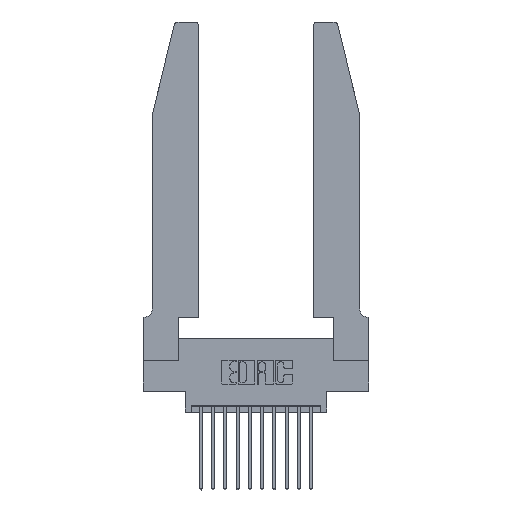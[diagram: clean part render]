
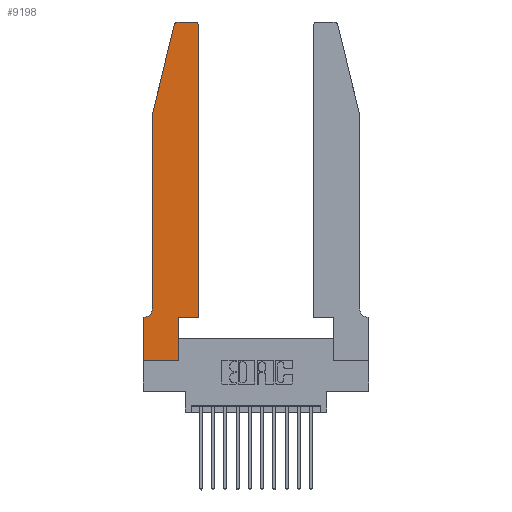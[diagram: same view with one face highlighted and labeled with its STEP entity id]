
A CAD part, top view. The second image highlights one B-rep face of the part: STEP entity #9198.
In plain terms, the highlighted planar face has unit normal (0, 0, 1).
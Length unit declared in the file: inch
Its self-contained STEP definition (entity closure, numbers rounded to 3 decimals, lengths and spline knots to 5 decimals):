
#285 = CARTESIAN_POINT ( 'NONE',  ( 0.284, 2.72, 0.37 ) ) ;
#491 = CARTESIAN_POINT ( 'NONE',  ( 0.2605, 2.75, 0.37 ) ) ;
#730 = CIRCLE ( 'NONE', #12264, 0.03 ) ;
#994 = CARTESIAN_POINT ( 'NONE',  ( 0.0755, 2., 0.37 ) ) ;
#1283 = EDGE_CURVE ( 'NONE', #11578, #4585, #10848, .T. ) ;
#1331 = CARTESIAN_POINT ( 'NONE',  ( 0.284, 2.75, 0.37 ) ) ;
#1340 = CIRCLE ( 'NONE', #5759, 0.07 ) ;
#1403 = VERTEX_POINT ( 'NONE', #15737 ) ;
#1602 = DIRECTION ( 'NONE',  ( 1., 0., 0. ) ) ;
#1617 = EDGE_CURVE ( 'NONE', #6264, #10600, #730, .T. ) ;
#1886 = ORIENTED_EDGE ( 'NONE', *, *, #4167, .T. ) ;
#1912 = LINE ( 'NONE', #8963, #12431 ) ;
#2145 = EDGE_CURVE ( 'NONE', #4585, #13388, #1340, .T. ) ;
#2500 = DIRECTION ( 'NONE',  ( -0.239, -0.971, 0. ) ) ;
#2505 = ORIENTED_EDGE ( 'NONE', *, *, #2699, .T. ) ;
#2699 = EDGE_CURVE ( 'NONE', #11066, #11127, #12644, .T. ) ;
#2708 = DIRECTION ( 'NONE',  ( 0., -1., 0. ) ) ;
#2823 = CARTESIAN_POINT ( 'NONE',  ( 0.4205, 2.75, 0.37 ) ) ;
#3012 = VECTOR ( 'NONE', #8688, 39.37008 ) ;
#3456 = DIRECTION ( 'NONE',  ( 1., 0., 0. ) ) ;
#3475 = CARTESIAN_POINT ( 'NONE',  ( 0.4205, 2.72, 0.37 ) ) ;
#3590 = DIRECTION ( 'NONE',  ( 0., 0., 1. ) ) ;
#4015 = EDGE_CURVE ( 'NONE', #1403, #5739, #5811, .T. ) ;
#4167 = EDGE_CURVE ( 'NONE', #10600, #11578, #1912, .T. ) ;
#4585 = VERTEX_POINT ( 'NONE', #6117 ) ;
#4599 = EDGE_CURVE ( 'NONE', #16292, #9981, #14475, .T. ) ;
#4806 = DIRECTION ( 'NONE',  ( 0., 0., -1. ) ) ;
#5260 = FACE_OUTER_BOUND ( 'NONE', #16275, .T. ) ;
#5327 = CARTESIAN_POINT ( 'NONE',  ( 0.0755, 0.35, 0.37 ) ) ;
#5358 = AXIS2_PLACEMENT_3D ( 'NONE', #3475, #3590, #15305 ) ;
#5403 = VECTOR ( 'NONE', #5986, 39.37008 ) ;
#5739 = VERTEX_POINT ( 'NONE', #8305 ) ;
#5759 = AXIS2_PLACEMENT_3D ( 'NONE', #11400, #4806, #10040 ) ;
#5766 = VECTOR ( 'NONE', #12237, 39.37008 ) ;
#5811 = LINE ( 'NONE', #11386, #12211 ) ;
#5820 = CIRCLE ( 'NONE', #5358, 0.03 ) ;
#5929 = DIRECTION ( 'NONE',  ( 1., 0., 0. ) ) ;
#5986 = DIRECTION ( 'NONE',  ( 0., 1., 0. ) ) ;
#6117 = CARTESIAN_POINT ( 'NONE',  ( 0.0755, 0.42, 0.37 ) ) ;
#6166 = PLANE ( 'NONE',  #10211 ) ;
#6233 = VERTEX_POINT ( 'NONE', #2823 ) ;
#6264 = VERTEX_POINT ( 'NONE', #1331 ) ;
#6312 = ORIENTED_EDGE ( 'NONE', *, *, #1617, .T. ) ;
#6498 = EDGE_CURVE ( 'NONE', #9981, #1403, #16035, .T. ) ;
#6626 = DIRECTION ( 'NONE',  ( 0., 1., 0. ) ) ;
#6808 = CARTESIAN_POINT ( 'NONE',  ( 0.2865, 0.35, 0.37 ) ) ;
#7047 = ORIENTED_EDGE ( 'NONE', *, *, #4599, .T. ) ;
#7128 = DIRECTION ( 'NONE',  ( 0., -1., 0. ) ) ;
#7188 = CARTESIAN_POINT ( 'NONE',  ( 0., 0., 0.37 ) ) ;
#7495 = CARTESIAN_POINT ( 'NONE',  ( 0., 0., 0.37 ) ) ;
#8305 = CARTESIAN_POINT ( 'NONE',  ( 0.4505, 2.72, 0.37 ) ) ;
#8359 = ORIENTED_EDGE ( 'NONE', *, *, #4015, .T. ) ;
#8688 = DIRECTION ( 'NONE',  ( 1., 0., 0. ) ) ;
#8821 = CARTESIAN_POINT ( 'NONE',  ( 0.0055, 0.35, 0.37 ) ) ;
#8963 = CARTESIAN_POINT ( 'NONE',  ( 0.0755, 2., 0.37 ) ) ;
#9198 = ADVANCED_FACE ( 'NONE', ( #5260 ), #6166, .T. ) ;
#9345 = CARTESIAN_POINT ( 'NONE',  ( 0., 0., 0.37 ) ) ;
#9489 = DIRECTION ( 'NONE',  ( 0., 0., 1. ) ) ;
#9929 = ORIENTED_EDGE ( 'NONE', *, *, #1283, .T. ) ;
#9981 = VERTEX_POINT ( 'NONE', #13438 ) ;
#10030 = DIRECTION ( 'NONE',  ( 0., 0., 1. ) ) ;
#10040 = DIRECTION ( 'NONE',  ( -1., 0., 0. ) ) ;
#10211 = AXIS2_PLACEMENT_3D ( 'NONE', #11333, #10030, #3456 ) ;
#10441 = LINE ( 'NONE', #5327, #11683 ) ;
#10454 = EDGE_CURVE ( 'NONE', #5739, #6233, #5820, .T. ) ;
#10600 = VERTEX_POINT ( 'NONE', #13426 ) ;
#10695 = ORIENTED_EDGE ( 'NONE', *, *, #13991, .T. ) ;
#10848 = LINE ( 'NONE', #994, #11867 ) ;
#11066 = VERTEX_POINT ( 'NONE', #16990 ) ;
#11127 = VERTEX_POINT ( 'NONE', #9345 ) ;
#11333 = CARTESIAN_POINT ( 'NONE',  ( 0., 0.35, 0.37 ) ) ;
#11386 = CARTESIAN_POINT ( 'NONE',  ( 0.4505, 0.35, 0.37 ) ) ;
#11400 = CARTESIAN_POINT ( 'NONE',  ( 0.0055, 0.42, 0.37 ) ) ;
#11578 = VERTEX_POINT ( 'NONE', #12691 ) ;
#11610 = VECTOR ( 'NONE', #7128, 39.37008 ) ;
#11683 = VECTOR ( 'NONE', #15712, 39.37008 ) ;
#11867 = VECTOR ( 'NONE', #2708, 39.37008 ) ;
#12211 = VECTOR ( 'NONE', #6626, 39.37008 ) ;
#12237 = DIRECTION ( 'NONE',  ( -1., 0., 0. ) ) ;
#12264 = AXIS2_PLACEMENT_3D ( 'NONE', #285, #9489, #1602 ) ;
#12431 = VECTOR ( 'NONE', #2500, 39.37008 ) ;
#12644 = LINE ( 'NONE', #7188, #11610 ) ;
#12691 = CARTESIAN_POINT ( 'NONE',  ( 0.0755, 2., 0.37 ) ) ;
#12925 = CARTESIAN_POINT ( 'NONE',  ( 0.2865, 0., 0.37 ) ) ;
#13388 = VERTEX_POINT ( 'NONE', #8821 ) ;
#13426 = CARTESIAN_POINT ( 'NONE',  ( 0.25487, 2.72718, 0.37 ) ) ;
#13438 = CARTESIAN_POINT ( 'NONE',  ( 0.2865, 0.35, 0.37 ) ) ;
#13842 = CARTESIAN_POINT ( 'NONE',  ( 0.4505, 0.35, 0.37 ) ) ;
#13893 = ORIENTED_EDGE ( 'NONE', *, *, #10454, .T. ) ;
#13960 = LINE ( 'NONE', #7495, #3012 ) ;
#13991 = EDGE_CURVE ( 'NONE', #11127, #16292, #13960, .T. ) ;
#14475 = LINE ( 'NONE', #6808, #5403 ) ;
#14813 = ORIENTED_EDGE ( 'NONE', *, *, #14979, .T. ) ;
#14979 = EDGE_CURVE ( 'NONE', #6233, #6264, #15825, .T. ) ;
#15298 = ORIENTED_EDGE ( 'NONE', *, *, #2145, .T. ) ;
#15305 = DIRECTION ( 'NONE',  ( 1., 0., 0. ) ) ;
#15495 = ORIENTED_EDGE ( 'NONE', *, *, #6498, .T. ) ;
#15712 = DIRECTION ( 'NONE',  ( -1., 0., 0. ) ) ;
#15737 = CARTESIAN_POINT ( 'NONE',  ( 0.4505, 0.35, 0.37 ) ) ;
#15825 = LINE ( 'NONE', #491, #5766 ) ;
#16035 = LINE ( 'NONE', #13842, #16869 ) ;
#16275 = EDGE_LOOP ( 'NONE', ( #14813, #6312, #1886, #9929, #15298, #16457, #2505, #10695, #7047, #15495, #8359, #13893 ) ) ;
#16292 = VERTEX_POINT ( 'NONE', #12925 ) ;
#16402 = EDGE_CURVE ( 'NONE', #13388, #11066, #10441, .T. ) ;
#16457 = ORIENTED_EDGE ( 'NONE', *, *, #16402, .T. ) ;
#16869 = VECTOR ( 'NONE', #5929, 39.37008 ) ;
#16990 = CARTESIAN_POINT ( 'NONE',  ( 0., 0.35, 0.37 ) ) ;
